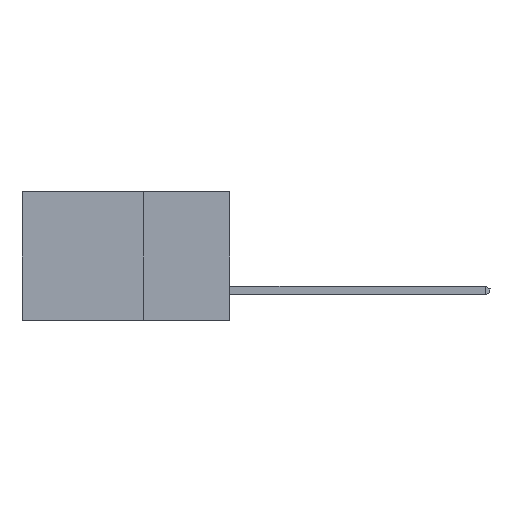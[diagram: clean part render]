
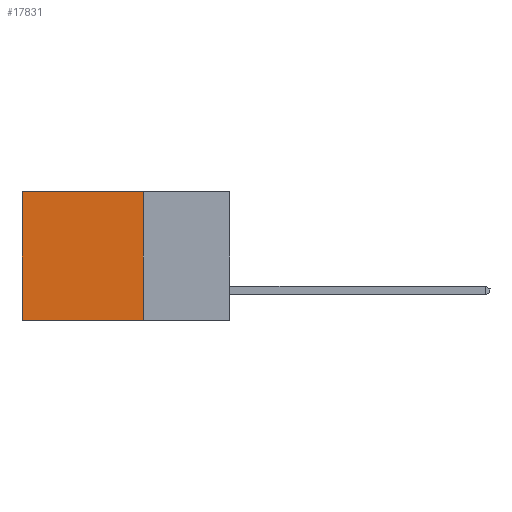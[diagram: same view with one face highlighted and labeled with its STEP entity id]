
A CAD part, left-side view. The second image highlights one B-rep face of the part: STEP entity #17831.
In plain terms, the highlighted planar face has unit normal (-1, 0, 0).
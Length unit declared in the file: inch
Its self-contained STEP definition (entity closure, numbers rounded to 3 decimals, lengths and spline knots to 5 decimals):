
#907 = PLANE ( 'NONE',  #949 ) ;
#949 = AXIS2_PLACEMENT_3D ( 'NONE', #8187, #15473, #6412 ) ;
#1622 = DIRECTION ( 'NONE',  ( 0., 1., 0. ) ) ;
#1968 = EDGE_LOOP ( 'NONE', ( #3608, #6948, #21247, #3829 ) ) ;
#3300 = EDGE_CURVE ( 'NONE', #12543, #12937, #22052, .T. ) ;
#3608 = ORIENTED_EDGE ( 'NONE', *, *, #11882, .T. ) ;
#3829 = ORIENTED_EDGE ( 'NONE', *, *, #3300, .T. ) ;
#5171 = EDGE_CURVE ( 'NONE', #12579, #16674, #20111, .T. ) ;
#6301 = LINE ( 'NONE', #8431, #22469 ) ;
#6412 = DIRECTION ( 'NONE',  ( 0., 0., -1. ) ) ;
#6948 = ORIENTED_EDGE ( 'NONE', *, *, #5171, .F. ) ;
#7159 = CARTESIAN_POINT ( 'NONE',  ( 0.2615, 0.25, 0. ) ) ;
#7612 = CARTESIAN_POINT ( 'NONE',  ( 0.2615, 0.25, 0. ) ) ;
#8187 = CARTESIAN_POINT ( 'NONE',  ( 0.2615, 0.25, -0.37 ) ) ;
#8431 = CARTESIAN_POINT ( 'NONE',  ( 0.2615, 0.25, -0.37 ) ) ;
#8818 = CARTESIAN_POINT ( 'NONE',  ( 0.2615, 0.25, -0.37 ) ) ;
#9249 = CARTESIAN_POINT ( 'NONE',  ( 0.2615, 0.6, 0. ) ) ;
#9960 = FACE_OUTER_BOUND ( 'NONE', #1968, .T. ) ;
#11672 = CARTESIAN_POINT ( 'NONE',  ( 0.2615, 0.6, -0.37 ) ) ;
#11882 = EDGE_CURVE ( 'NONE', #12937, #16674, #17645, .T. ) ;
#12543 = VERTEX_POINT ( 'NONE', #7159 ) ;
#12579 = VERTEX_POINT ( 'NONE', #8818 ) ;
#12937 = VERTEX_POINT ( 'NONE', #9249 ) ;
#13336 = DIRECTION ( 'NONE',  ( 0., 0., -1. ) ) ;
#15473 = DIRECTION ( 'NONE',  ( 1., 0., 0. ) ) ;
#16444 = DIRECTION ( 'NONE',  ( 0., 1., 0. ) ) ;
#16492 = CARTESIAN_POINT ( 'NONE',  ( 0.2615, 0.6, -0.37 ) ) ;
#16674 = VERTEX_POINT ( 'NONE', #16492 ) ;
#16691 = VECTOR ( 'NONE', #1622, 39.37008 ) ;
#16981 = VECTOR ( 'NONE', #16444, 39.37008 ) ;
#17586 = VECTOR ( 'NONE', #19090, 39.37008 ) ;
#17645 = LINE ( 'NONE', #11672, #17586 ) ;
#17831 = ADVANCED_FACE ( 'NONE', ( #9960 ), #907, .F. ) ;
#19090 = DIRECTION ( 'NONE',  ( 0., 0., -1. ) ) ;
#20111 = LINE ( 'NONE', #23451, #16691 ) ;
#21247 = ORIENTED_EDGE ( 'NONE', *, *, #22413, .F. ) ;
#22052 = LINE ( 'NONE', #7612, #16981 ) ;
#22413 = EDGE_CURVE ( 'NONE', #12543, #12579, #6301, .T. ) ;
#22469 = VECTOR ( 'NONE', #13336, 39.37008 ) ;
#23451 = CARTESIAN_POINT ( 'NONE',  ( 0.2615, 0.25, -0.37 ) ) ;
